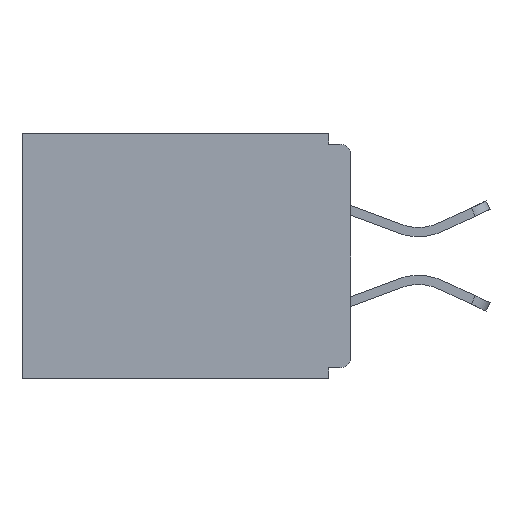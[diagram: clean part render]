
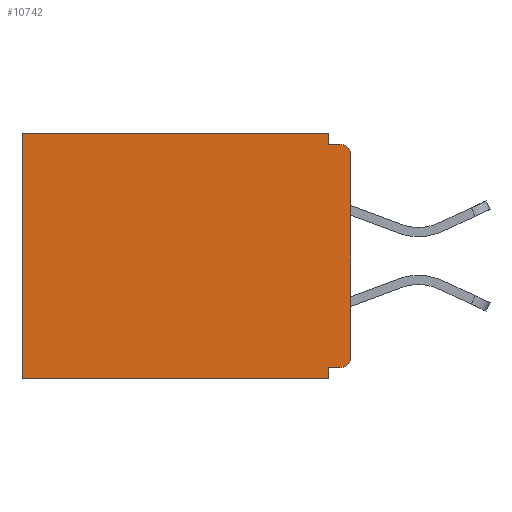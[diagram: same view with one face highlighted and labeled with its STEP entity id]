
A CAD part, left-side view. The second image highlights one B-rep face of the part: STEP entity #10742.
In plain terms, the highlighted planar face has unit normal (-1, 0, 0).
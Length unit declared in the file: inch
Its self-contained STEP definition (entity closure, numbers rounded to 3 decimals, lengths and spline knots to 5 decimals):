
#237 = ORIENTED_EDGE ( 'NONE', *, *, #8265, .T. ) ;
#271 = DIRECTION ( 'NONE',  ( 0., 0., -1. ) ) ;
#524 = ORIENTED_EDGE ( 'NONE', *, *, #9692, .F. ) ;
#612 = ORIENTED_EDGE ( 'NONE', *, *, #5912, .T. ) ;
#791 = ORIENTED_EDGE ( 'NONE', *, *, #14341, .T. ) ;
#1121 = PLANE ( 'NONE',  #7241 ) ;
#1162 = VECTOR ( 'NONE', #16126, 39.37008 ) ;
#1195 = CARTESIAN_POINT ( 'NONE',  ( 0.298, 0.031, -0.343 ) ) ;
#1244 = CIRCLE ( 'NONE', #2641, 0.015 ) ;
#1498 = VECTOR ( 'NONE', #271, 39.37008 ) ;
#1645 = LINE ( 'NONE', #13274, #1162 ) ;
#1675 = VERTEX_POINT ( 'NONE', #10379 ) ;
#2112 = EDGE_CURVE ( 'NONE', #16021, #12000, #9160, .T. ) ;
#2229 = LINE ( 'NONE', #2503, #3172 ) ;
#2503 = CARTESIAN_POINT ( 'NONE',  ( 0.298, 0.031, -0.343 ) ) ;
#2531 = EDGE_CURVE ( 'NONE', #3655, #12000, #16968, .T. ) ;
#2641 = AXIS2_PLACEMENT_3D ( 'NONE', #13426, #6274, #6462 ) ;
#2865 = LINE ( 'NONE', #6384, #8678 ) ;
#2898 = VECTOR ( 'NONE', #4156, 39.37008 ) ;
#2948 = CARTESIAN_POINT ( 'NONE',  ( 0.298, 0.46, -0.343 ) ) ;
#3172 = VECTOR ( 'NONE', #3977, 39.37008 ) ;
#3639 = LINE ( 'NONE', #12748, #15882 ) ;
#3655 = VERTEX_POINT ( 'NONE', #1195 ) ;
#3977 = DIRECTION ( 'NONE',  ( 0., 0., -1. ) ) ;
#4135 = DIRECTION ( 'NONE',  ( 0., 0., -1. ) ) ;
#4156 = DIRECTION ( 'NONE',  ( 0., 0., -1. ) ) ;
#4157 = ORIENTED_EDGE ( 'NONE', *, *, #2112, .T. ) ;
#4346 = CARTESIAN_POINT ( 'NONE',  ( 0.298, 0.031, -0.343 ) ) ;
#4438 = VERTEX_POINT ( 'NONE', #15223 ) ;
#4488 = DIRECTION ( 'NONE',  ( -1., 0., 0. ) ) ;
#4923 = DIRECTION ( 'NONE',  ( 0., -1., 0. ) ) ;
#5217 = CARTESIAN_POINT ( 'NONE',  ( 0.298, 0., -0.03 ) ) ;
#5378 = CARTESIAN_POINT ( 'NONE',  ( 0.298, 0.46, 0. ) ) ;
#5542 = VERTEX_POINT ( 'NONE', #14676 ) ;
#5761 = CARTESIAN_POINT ( 'NONE',  ( 0.298, 0.46, 0. ) ) ;
#5912 = EDGE_CURVE ( 'NONE', #16774, #15038, #16751, .T. ) ;
#6118 = AXIS2_PLACEMENT_3D ( 'NONE', #17432, #4488, #10148 ) ;
#6274 = DIRECTION ( 'NONE',  ( -1., 0., 0. ) ) ;
#6284 = EDGE_CURVE ( 'NONE', #1675, #12104, #2229, .T. ) ;
#6384 = CARTESIAN_POINT ( 'NONE',  ( 0.298, 0., -0.328 ) ) ;
#6462 = DIRECTION ( 'NONE',  ( 0., 0., -1. ) ) ;
#6511 = DIRECTION ( 'NONE',  ( 0., 1., 0. ) ) ;
#6815 = CARTESIAN_POINT ( 'NONE',  ( 0.298, 0., -0.343 ) ) ;
#7241 = AXIS2_PLACEMENT_3D ( 'NONE', #8240, #11114, #4135 ) ;
#8240 = CARTESIAN_POINT ( 'NONE',  ( 0.298, 0., 0. ) ) ;
#8265 = EDGE_CURVE ( 'NONE', #4438, #17403, #1244, .T. ) ;
#8678 = VECTOR ( 'NONE', #6511, 39.37008 ) ;
#9160 = LINE ( 'NONE', #5761, #2898 ) ;
#9299 = ORIENTED_EDGE ( 'NONE', *, *, #2531, .F. ) ;
#9355 = LINE ( 'NONE', #12037, #12271 ) ;
#9692 = EDGE_CURVE ( 'NONE', #12104, #15038, #9355, .T. ) ;
#10148 = DIRECTION ( 'NONE',  ( 0., 0., -1. ) ) ;
#10225 = EDGE_CURVE ( 'NONE', #5542, #3655, #14242, .T. ) ;
#10343 = EDGE_CURVE ( 'NONE', #4438, #5542, #2865, .T. ) ;
#10379 = CARTESIAN_POINT ( 'NONE',  ( 0.298, 0.031, 0. ) ) ;
#10742 = ADVANCED_FACE ( 'NONE', ( #14686 ), #1121, .F. ) ;
#11047 = CARTESIAN_POINT ( 'NONE',  ( 0.298, 0.031, -0.015 ) ) ;
#11114 = DIRECTION ( 'NONE',  ( 1., 0., 0. ) ) ;
#11144 = DIRECTION ( 'NONE',  ( 0., 1., 0. ) ) ;
#12000 = VERTEX_POINT ( 'NONE', #2948 ) ;
#12037 = CARTESIAN_POINT ( 'NONE',  ( 0.298, 0., -0.015 ) ) ;
#12104 = VERTEX_POINT ( 'NONE', #11047 ) ;
#12271 = VECTOR ( 'NONE', #4923, 39.37008 ) ;
#12748 = CARTESIAN_POINT ( 'NONE',  ( 0.298, 0., 0. ) ) ;
#13208 = EDGE_CURVE ( 'NONE', #16774, #17403, #1645, .T. ) ;
#13274 = CARTESIAN_POINT ( 'NONE',  ( 0.298, 0., 0. ) ) ;
#13426 = CARTESIAN_POINT ( 'NONE',  ( 0.298, 0.015, -0.313 ) ) ;
#14242 = LINE ( 'NONE', #4346, #1498 ) ;
#14341 = EDGE_CURVE ( 'NONE', #1675, #16021, #3639, .T. ) ;
#14613 = ORIENTED_EDGE ( 'NONE', *, *, #13208, .F. ) ;
#14676 = CARTESIAN_POINT ( 'NONE',  ( 0.298, 0.031, -0.328 ) ) ;
#14686 = FACE_OUTER_BOUND ( 'NONE', #14819, .T. ) ;
#14819 = EDGE_LOOP ( 'NONE', ( #612, #524, #18486, #791, #4157, #9299, #16379, #17579, #237, #14613 ) ) ;
#14929 = CARTESIAN_POINT ( 'NONE',  ( 0.298, 0., -0.313 ) ) ;
#15038 = VERTEX_POINT ( 'NONE', #15418 ) ;
#15223 = CARTESIAN_POINT ( 'NONE',  ( 0.298, 0.015, -0.328 ) ) ;
#15418 = CARTESIAN_POINT ( 'NONE',  ( 0.298, 0.015, -0.015 ) ) ;
#15611 = VECTOR ( 'NONE', #16757, 39.37008 ) ;
#15882 = VECTOR ( 'NONE', #11144, 39.37008 ) ;
#16021 = VERTEX_POINT ( 'NONE', #5378 ) ;
#16126 = DIRECTION ( 'NONE',  ( 0., 0., -1. ) ) ;
#16379 = ORIENTED_EDGE ( 'NONE', *, *, #10225, .F. ) ;
#16751 = CIRCLE ( 'NONE', #6118, 0.015 ) ;
#16757 = DIRECTION ( 'NONE',  ( 0., 1., 0. ) ) ;
#16774 = VERTEX_POINT ( 'NONE', #5217 ) ;
#16968 = LINE ( 'NONE', #6815, #15611 ) ;
#17403 = VERTEX_POINT ( 'NONE', #14929 ) ;
#17432 = CARTESIAN_POINT ( 'NONE',  ( 0.298, 0.015, -0.03 ) ) ;
#17579 = ORIENTED_EDGE ( 'NONE', *, *, #10343, .F. ) ;
#18486 = ORIENTED_EDGE ( 'NONE', *, *, #6284, .F. ) ;
